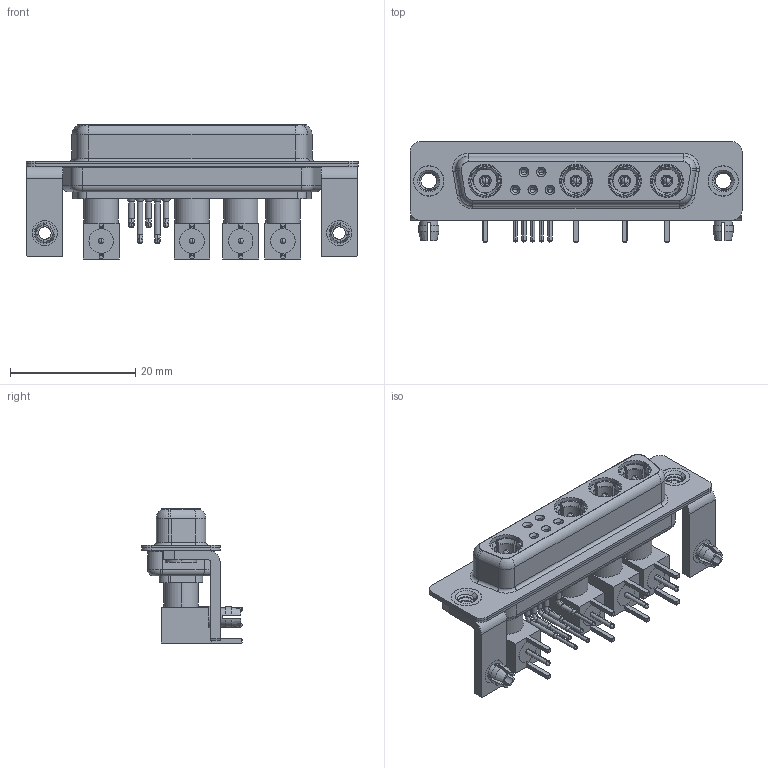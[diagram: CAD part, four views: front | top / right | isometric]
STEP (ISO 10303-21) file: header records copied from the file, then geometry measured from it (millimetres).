
FILE_DESCRIPTION (( 'STEP AP203' ), '1' );
FILE_NAME ('630-9W4-240-5TB.STEP', '2022-06-01T05:30:15', ( '' ), ( '' ), 'SwSTEP 2.0', 'SolidWorks 2020', '' );
FILE_SCHEMA (( 'CONFIG_CONTROL_DESIGN' ));
Length unit declared in the file: millimetre
Products named in the file (19): 630Combo Contact Row 1; Pin_RA; Co-Ax Plug Assy_RA; 630Combo Contact Row 2; 630Combo Stabilizer Bracket; 630Combo Shell Front_25 Contacts; 630Combo Threaded Rivet_B; Insulator RA Pin; 630Combo Housing_9W4; 630Combo Board Lock; 630-9W4-240-5TB; 630Combo Shell Rear_25 Contacts; Co-Ax Plug_RA PC Tail; Insulator Pin_Straight PC Tail; Locking Collar; RA Back Shell
Assembly tree (42 placements, depth 3):
  630-9W4-240-5TB
    630Combo Housing_9W4
    630Combo Shell Front_25 Contacts
    630Combo Shell Rear_25 Contacts
    630Combo Threaded Rivet_B  x2
    630Combo Stabilizer Bracket  x2
    630Combo Board Lock  x2
    Co-Ax Plug Assy_RA
      Co-Ax Plug_RA PC Tail
      Insulator Pin_Straight PC Tail
      Pin_RA
      Locking Collar
      RA Back Shell
      Insulator RA Pin
    Co-Ax Plug Assy_RA
      Co-Ax Plug_RA PC Tail
      Insulator Pin_Straight PC Tail
      Pin_RA
      Locking Collar
      RA Back Shell
      Insulator RA Pin
    Co-Ax Plug Assy_RA
      Co-Ax Plug_RA PC Tail
      Insulator Pin_Straight PC Tail
      Pin_RA
      Locking Collar
      RA Back Shell
      Insulator RA Pin
    Co-Ax Plug Assy_RA
      Co-Ax Plug_RA PC Tail
      Insulator Pin_Straight PC Tail
      Pin_RA
      Locking Collar
      RA Back Shell
      Insulator RA Pin
    630Combo Contact Row 1  x2
    630Combo Contact Row 2  x3
Bounding box: 53.05 x 16 x 21.41 mm (x, y, z)
Volume: 4984.3 mm3; surface area: 12129.8 mm2
Topology: 38 solids, 38 shells, 1346 faces, 3308 edges, 2082 vertices
Faces by surface type: cylinder 562, plane 478, cone 179, torus 81, bspline 30, sphere 16
Entity records: 23505 total; most frequent: CARTESIAN_POINT 5279, DIRECTION 3533, ORIENTED_EDGE 3094, EDGE_CURVE 1547, AXIS2_PLACEMENT_3D 1429, VERTEX_POINT 985, CIRCLE 753, EDGE_LOOP 734
